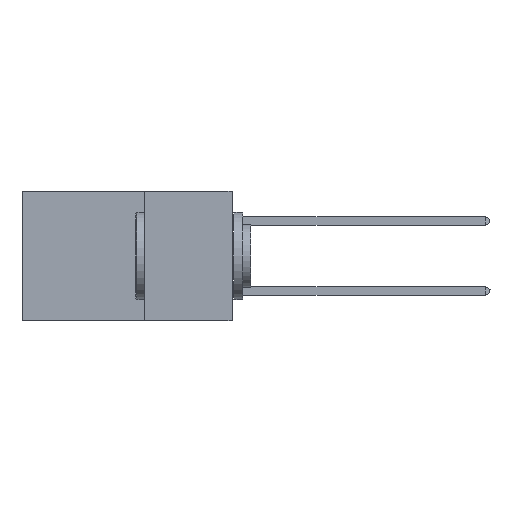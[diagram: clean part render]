
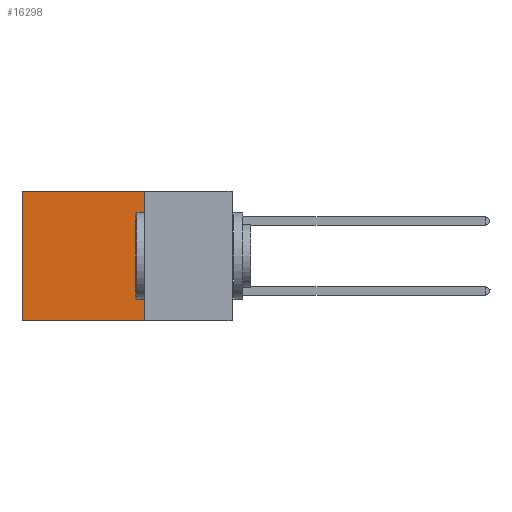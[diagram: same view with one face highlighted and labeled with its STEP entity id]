
A CAD part, left-side view. The second image highlights one B-rep face of the part: STEP entity #16298.
In plain terms, the highlighted planar face has unit normal (-1, 0, 0).
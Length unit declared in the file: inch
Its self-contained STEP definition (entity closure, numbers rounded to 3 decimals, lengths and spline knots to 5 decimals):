
#716 = ORIENTED_EDGE ( 'NONE', *, *, #25369, .F. ) ;
#765 = VECTOR ( 'NONE', #4920, 39.37008 ) ;
#816 = VERTEX_POINT ( 'NONE', #13134 ) ;
#1863 = CARTESIAN_POINT ( 'NONE',  ( 0.2875, 0.25, -0.37 ) ) ;
#2359 = CARTESIAN_POINT ( 'NONE',  ( 0.2875, 0.6, 0. ) ) ;
#2990 = DIRECTION ( 'NONE',  ( 0., 1., 0. ) ) ;
#4267 = LINE ( 'NONE', #24361, #18668 ) ;
#4447 = ORIENTED_EDGE ( 'NONE', *, *, #15625, .T. ) ;
#4920 = DIRECTION ( 'NONE',  ( 0., 0., -1. ) ) ;
#6907 = CARTESIAN_POINT ( 'NONE',  ( 0.2875, 0.25, 0. ) ) ;
#8522 = LINE ( 'NONE', #36102, #765 ) ;
#8821 = LINE ( 'NONE', #2359, #36265 ) ;
#10184 = LINE ( 'NONE', #23040, #31903 ) ;
#12851 = ORIENTED_EDGE ( 'NONE', *, *, #29873, .F. ) ;
#13134 = CARTESIAN_POINT ( 'NONE',  ( 0.2875, 0.6, -0.37 ) ) ;
#14130 = DIRECTION ( 'NONE',  ( 1., 0., 0. ) ) ;
#15625 = EDGE_CURVE ( 'NONE', #22098, #816, #8821, .T. ) ;
#15772 = EDGE_CURVE ( 'NONE', #29012, #22098, #10184, .T. ) ;
#16298 = ADVANCED_FACE ( 'NONE', ( #19922 ), #28195, .F. ) ;
#18668 = VECTOR ( 'NONE', #35515, 39.37008 ) ;
#19922 = FACE_OUTER_BOUND ( 'NONE', #30013, .T. ) ;
#22098 = VERTEX_POINT ( 'NONE', #27380 ) ;
#22438 = DIRECTION ( 'NONE',  ( 0., 0., -1. ) ) ;
#23040 = CARTESIAN_POINT ( 'NONE',  ( 0.2875, 0.25, 0. ) ) ;
#24361 = CARTESIAN_POINT ( 'NONE',  ( 0.2875, 0.25, -0.37 ) ) ;
#25369 = EDGE_CURVE ( 'NONE', #35913, #816, #4267, .T. ) ;
#27380 = CARTESIAN_POINT ( 'NONE',  ( 0.2875, 0.6, 0. ) ) ;
#28195 = PLANE ( 'NONE',  #35073 ) ;
#29012 = VERTEX_POINT ( 'NONE', #6907 ) ;
#29193 = ORIENTED_EDGE ( 'NONE', *, *, #15772, .T. ) ;
#29873 = EDGE_CURVE ( 'NONE', #29012, #35913, #8522, .T. ) ;
#30013 = EDGE_LOOP ( 'NONE', ( #4447, #716, #12851, #29193 ) ) ;
#31029 = CARTESIAN_POINT ( 'NONE',  ( 0.2875, 0.25, 0. ) ) ;
#31903 = VECTOR ( 'NONE', #2990, 39.37008 ) ;
#33856 = DIRECTION ( 'NONE',  ( 0., 0., -1. ) ) ;
#35073 = AXIS2_PLACEMENT_3D ( 'NONE', #31029, #14130, #33856 ) ;
#35515 = DIRECTION ( 'NONE',  ( 0., 1., 0. ) ) ;
#35913 = VERTEX_POINT ( 'NONE', #1863 ) ;
#36102 = CARTESIAN_POINT ( 'NONE',  ( 0.2875, 0.25, 0. ) ) ;
#36265 = VECTOR ( 'NONE', #22438, 39.37008 ) ;
